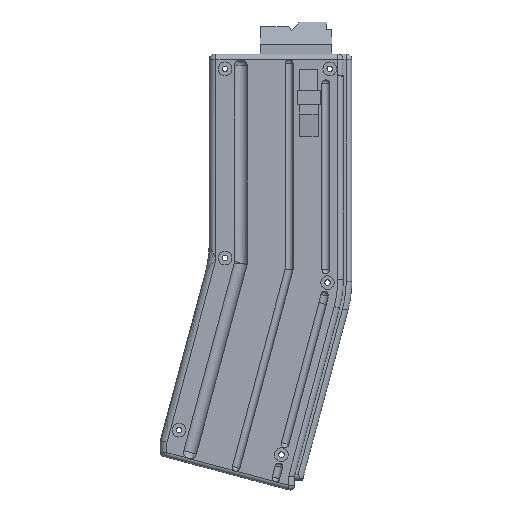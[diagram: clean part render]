
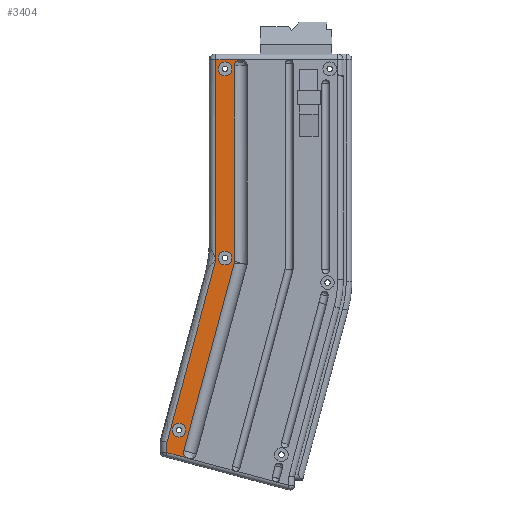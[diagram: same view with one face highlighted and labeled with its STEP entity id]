
A CAD part, front view. The second image highlights one B-rep face of the part: STEP entity #3404.
In plain terms, the highlighted planar face has unit normal (0, -1, 0).
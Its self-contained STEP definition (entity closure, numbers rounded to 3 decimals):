
#23=FACE_BOUND('',#695,.T.);
#24=FACE_BOUND('',#696,.T.);
#25=FACE_BOUND('',#697,.T.);
#118=B_SPLINE_CURVE_WITH_KNOTS('',3,(#5828,#5829,#5830,#5831,#5832,#5833,
#5834,#5835,#5836,#5837,#5838,#5839),.UNSPECIFIED.,.F.,.F.,(4,2,2,2,2,4),
(0.,0.112,0.224,0.335,0.439,
0.44),.UNSPECIFIED.);
#120=B_SPLINE_CURVE_WITH_KNOTS('',3,(#5972,#5973,#5974,#5975,#5976,#5977,
#5978,#5979,#5980,#5981,#5982,#5983),.UNSPECIFIED.,.F.,.F.,(4,2,2,2,2,4),
(-0.001,0.,0.105,0.216,0.327,
0.439),.UNSPECIFIED.);
#122=B_SPLINE_CURVE_WITH_KNOTS('',3,(#6041,#6042,#6043,#6044,#6045,#6046,
#6047,#6048,#6049,#6050,#6051,#6052,#6053),.UNSPECIFIED.,.F.,.F.,(4,3,3,
3,4),(0.,0.024,0.037,0.061,0.073),
 .UNSPECIFIED.);
#352=CIRCLE('',#3661,3.075);
#353=CIRCLE('',#3662,3.075);
#354=CIRCLE('',#3663,3.075);
#482=FACE_OUTER_BOUND('',#694,.T.);
#694=EDGE_LOOP('',(#2483,#2484,#2485,#2486,#2487,#2488,#2489,#2490,#2491,
#2492,#2493));
#695=EDGE_LOOP('',(#2494));
#696=EDGE_LOOP('',(#2495));
#697=EDGE_LOOP('',(#2496));
#901=LINE('',#5512,#1146);
#925=LINE('',#5858,#1170);
#927=LINE('',#5998,#1172);
#928=LINE('',#6056,#1173);
#929=LINE('',#6058,#1174);
#930=LINE('',#6060,#1175);
#931=LINE('',#6062,#1176);
#932=LINE('',#6063,#1177);
#1146=VECTOR('',#4050,10.);
#1170=VECTOR('',#4108,10.);
#1172=VECTOR('',#4112,10.);
#1173=VECTOR('',#4119,10.);
#1174=VECTOR('',#4120,10.);
#1175=VECTOR('',#4121,10.);
#1176=VECTOR('',#4122,10.);
#1177=VECTOR('',#4123,10.);
#1425=VERTEX_POINT('',#5509);
#1426=VERTEX_POINT('',#5511);
#1460=VERTEX_POINT('',#5827);
#1462=VERTEX_POINT('',#5856);
#1463=VERTEX_POINT('',#5969);
#1464=VERTEX_POINT('',#5971);
#1465=VERTEX_POINT('',#5997);
#1466=VERTEX_POINT('',#6055);
#1467=VERTEX_POINT('',#6057);
#1468=VERTEX_POINT('',#6059);
#1469=VERTEX_POINT('',#6061);
#1470=VERTEX_POINT('',#6064);
#1471=VERTEX_POINT('',#6066);
#1472=VERTEX_POINT('',#6068);
#1792=EDGE_CURVE('',#1425,#1426,#901,.T.);
#1833=EDGE_CURVE('',#1425,#1460,#118,.F.);
#1837=EDGE_CURVE('',#1460,#1462,#925,.T.);
#1839=EDGE_CURVE('',#1463,#1464,#120,.T.);
#1841=EDGE_CURVE('',#1465,#1464,#927,.T.);
#1844=EDGE_CURVE('',#1465,#1462,#122,.T.);
#1845=EDGE_CURVE('',#1466,#1463,#928,.T.);
#1846=EDGE_CURVE('',#1467,#1466,#929,.T.);
#1847=EDGE_CURVE('',#1467,#1468,#930,.T.);
#1848=EDGE_CURVE('',#1469,#1468,#931,.T.);
#1849=EDGE_CURVE('',#1426,#1469,#932,.T.);
#1850=EDGE_CURVE('',#1470,#1470,#352,.T.);
#1851=EDGE_CURVE('',#1471,#1471,#353,.T.);
#1852=EDGE_CURVE('',#1472,#1472,#354,.T.);
#2483=ORIENTED_EDGE('',*,*,#1844,.F.);
#2484=ORIENTED_EDGE('',*,*,#1841,.T.);
#2485=ORIENTED_EDGE('',*,*,#1839,.F.);
#2486=ORIENTED_EDGE('',*,*,#1845,.F.);
#2487=ORIENTED_EDGE('',*,*,#1846,.F.);
#2488=ORIENTED_EDGE('',*,*,#1847,.T.);
#2489=ORIENTED_EDGE('',*,*,#1848,.F.);
#2490=ORIENTED_EDGE('',*,*,#1849,.F.);
#2491=ORIENTED_EDGE('',*,*,#1792,.F.);
#2492=ORIENTED_EDGE('',*,*,#1833,.T.);
#2493=ORIENTED_EDGE('',*,*,#1837,.T.);
#2494=ORIENTED_EDGE('',*,*,#1850,.T.);
#2495=ORIENTED_EDGE('',*,*,#1851,.T.);
#2496=ORIENTED_EDGE('',*,*,#1852,.T.);
#3286=PLANE('',#3660);
#3404=ADVANCED_FACE('',(#482,#23,#24,#25),#3286,.T.);
#3660=AXIS2_PLACEMENT_3D('',#6054,#4117,#4118);
#3661=AXIS2_PLACEMENT_3D('',#6065,#4124,#4125);
#3662=AXIS2_PLACEMENT_3D('',#6067,#4126,#4127);
#3663=AXIS2_PLACEMENT_3D('',#6069,#4128,#4129);
#4050=DIRECTION('',(-0.966,0.,0.259));
#4108=DIRECTION('',(0.259,0.,0.966));
#4112=DIRECTION('',(0.,0.,1.));
#4117=DIRECTION('center_axis',(0.,-1.,0.));
#4118=DIRECTION('ref_axis',(1.,0.,0.));
#4119=DIRECTION('',(1.,0.,0.));
#4120=DIRECTION('',(0.,0.,1.));
#4121=DIRECTION('',(-0.259,0.,-0.966));
#4122=DIRECTION('',(0.966,0.,-0.259));
#4123=DIRECTION('',(0.,0.,1.));
#4124=DIRECTION('center_axis',(0.,1.,0.));
#4125=DIRECTION('ref_axis',(1.,0.,0.));
#4126=DIRECTION('center_axis',(0.,1.,0.));
#4127=DIRECTION('ref_axis',(1.,0.,0.));
#4128=DIRECTION('center_axis',(0.,1.,0.));
#4129=DIRECTION('ref_axis',(1.,0.,0.));
#5509=CARTESIAN_POINT('',(326.692,-38.877,-148.043));
#5511=CARTESIAN_POINT('',(317.124,-38.877,-145.479));
#5512=CARTESIAN_POINT('',(332.652,-38.877,-149.64));
#5827=CARTESIAN_POINT('',(324.724,-38.877,-144.621));
#5828=CARTESIAN_POINT('Ctrl Pts',(324.724,-38.877,-144.621));
#5829=CARTESIAN_POINT('Ctrl Pts',(324.627,-38.877,-144.982));
#5830=CARTESIAN_POINT('Ctrl Pts',(324.603,-38.877,-145.36));
#5831=CARTESIAN_POINT('Ctrl Pts',(324.705,-38.877,-146.098));
#5832=CARTESIAN_POINT('Ctrl Pts',(324.829,-38.877,-146.452));
#5833=CARTESIAN_POINT('Ctrl Pts',(325.206,-38.877,-147.09));
#5834=CARTESIAN_POINT('Ctrl Pts',(325.456,-38.877,-147.367));
#5835=CARTESIAN_POINT('Ctrl Pts',(326.033,-38.877,-147.796));
#5836=CARTESIAN_POINT('Ctrl Pts',(326.349,-38.877,-147.95));
#5837=CARTESIAN_POINT('Ctrl Pts',(326.688,-38.877,-148.041));
#5838=CARTESIAN_POINT('Ctrl Pts',(326.69,-38.877,-148.042));
#5839=CARTESIAN_POINT('Ctrl Pts',(326.692,-38.877,-148.043));
#5856=CARTESIAN_POINT('',(347.308,-38.877,-60.335));
#5858=CARTESIAN_POINT('',(324.,-38.877,-147.321));
#5969=CARTESIAN_POINT('',(350.191,-38.877,30.987));
#5971=CARTESIAN_POINT('',(347.403,-38.877,28.191));
#5972=CARTESIAN_POINT('Ctrl Pts',(350.191,-38.877,30.987));
#5973=CARTESIAN_POINT('Ctrl Pts',(350.188,-38.877,30.987));
#5974=CARTESIAN_POINT('Ctrl Pts',(350.186,-38.877,30.987));
#5975=CARTESIAN_POINT('Ctrl Pts',(349.835,-38.877,30.986));
#5976=CARTESIAN_POINT('Ctrl Pts',(349.49,-38.877,30.919));
#5977=CARTESIAN_POINT('Ctrl Pts',(348.822,-38.877,30.654));
#5978=CARTESIAN_POINT('Ctrl Pts',(348.508,-38.877,30.451));
#5979=CARTESIAN_POINT('Ctrl Pts',(347.979,-38.877,29.933));
#5980=CARTESIAN_POINT('Ctrl Pts',(347.768,-38.877,29.623));
#5981=CARTESIAN_POINT('Ctrl Pts',(347.478,-38.877,28.936));
#5982=CARTESIAN_POINT('Ctrl Pts',(347.403,-38.877,28.565));
#5983=CARTESIAN_POINT('Ctrl Pts',(347.403,-38.877,28.191));
#5997=CARTESIAN_POINT('',(347.403,-38.877,-59.611));
#5998=CARTESIAN_POINT('',(347.403,-38.877,-60.362));
#6041=CARTESIAN_POINT('Ctrl Pts',(347.403,-38.877,-59.611));
#6042=CARTESIAN_POINT('Ctrl Pts',(347.403,-38.877,-59.692));
#6043=CARTESIAN_POINT('Ctrl Pts',(347.4,-38.877,-59.773));
#6044=CARTESIAN_POINT('Ctrl Pts',(347.393,-38.877,-59.853));
#6045=CARTESIAN_POINT('Ctrl Pts',(347.389,-38.877,-59.894));
#6046=CARTESIAN_POINT('Ctrl Pts',(347.385,-38.877,-59.935));
#6047=CARTESIAN_POINT('Ctrl Pts',(347.379,-38.877,-59.976));
#6048=CARTESIAN_POINT('Ctrl Pts',(347.369,-38.877,-60.056));
#6049=CARTESIAN_POINT('Ctrl Pts',(347.355,-38.877,-60.136));
#6050=CARTESIAN_POINT('Ctrl Pts',(347.337,-38.877,-60.215));
#6051=CARTESIAN_POINT('Ctrl Pts',(347.329,-38.877,-60.255));
#6052=CARTESIAN_POINT('Ctrl Pts',(347.319,-38.877,-60.295));
#6053=CARTESIAN_POINT('Ctrl Pts',(347.308,-38.877,-60.335));
#6054=CARTESIAN_POINT('Origin',(356.451,-38.877,-60.928));
#6055=CARTESIAN_POINT('',(339.124,-38.877,30.987));
#6056=CARTESIAN_POINT('',(372.807,-38.877,30.987));
#6057=CARTESIAN_POINT('',(339.124,-38.877,-58.889));
#6058=CARTESIAN_POINT('',(339.124,-38.877,-60.891));
#6059=CARTESIAN_POINT('',(317.15,-38.877,-140.896));
#6060=CARTESIAN_POINT('',(339.124,-38.877,-58.889));
#6061=CARTESIAN_POINT('',(317.124,-38.877,-140.889));
#6062=CARTESIAN_POINT('',(337.867,-38.877,-146.447));
#6063=CARTESIAN_POINT('',(317.124,-38.877,-142.891));
#6064=CARTESIAN_POINT('',(340.168,-38.877,-58.134));
#6065=CARTESIAN_POINT('Origin',(343.243,-38.877,-58.134));
#6066=CARTESIAN_POINT('',(340.168,-38.877,26.866));
#6067=CARTESIAN_POINT('Origin',(343.243,-38.877,26.866));
#6068=CARTESIAN_POINT('',(319.462,-38.877,-135.408));
#6069=CARTESIAN_POINT('Origin',(322.537,-38.877,-135.408));
